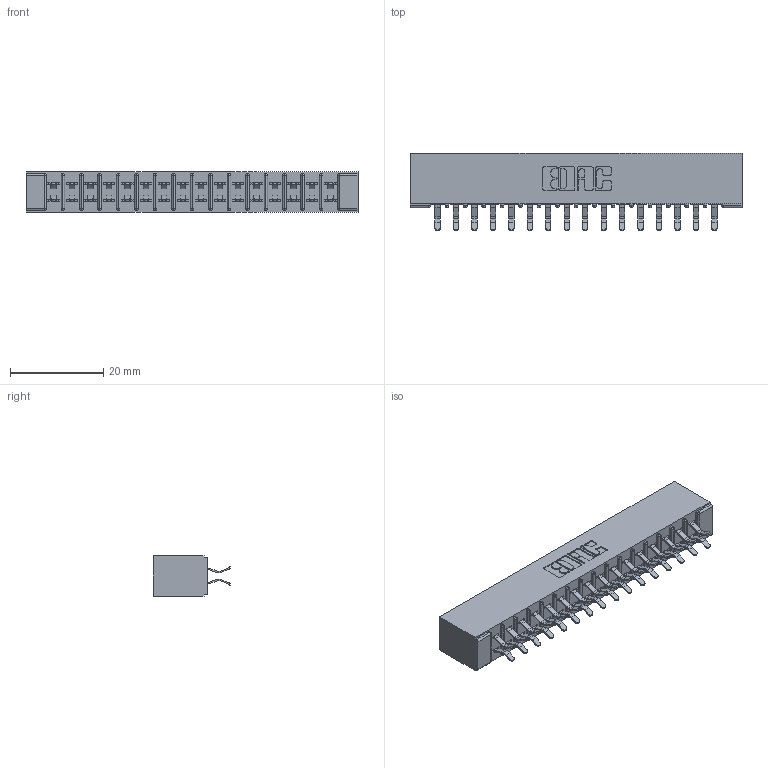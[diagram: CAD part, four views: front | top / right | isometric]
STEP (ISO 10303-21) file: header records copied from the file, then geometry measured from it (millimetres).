
FILE_DESCRIPTION (( 'STEP AP203' ), '1' );
FILE_NAME ('315-032-556-201.STEP', '2019-09-10T15:44:33', ( '' ), ( '' ), 'SwSTEP 2.0', 'SolidWorks 2016', '' );
FILE_SCHEMA (( 'CONFIG_CONTROL_DESIGN' ));
Length unit declared in the file: inch
Products named in the file (3): 305-290-001_556; 315-032-556-201; 305 Part_No Mounting
Assembly tree (33 placements, depth 2):
  315-032-556-201
    305 Part_No Mounting
    305-290-001_556  x32
Bounding box: 71.27 x 16.64 x 8.71 mm (x, y, z)
Volume: 4669 mm3; surface area: 9029.4 mm2
Topology: 33 solids, 33 shells, 1900 faces, 5460 edges, 3552 vertices
Faces by surface type: plane 1056, cylinder 780, sphere 64
Entity records: 20433 total; most frequent: CARTESIAN_POINT 3382, ORIENTED_EDGE 3352, DIRECTION 3294, EDGE_CURVE 1676, VECTOR 1326, LINE 1326, VERTEX_POINT 1072, AXIS2_PLACEMENT_3D 984
